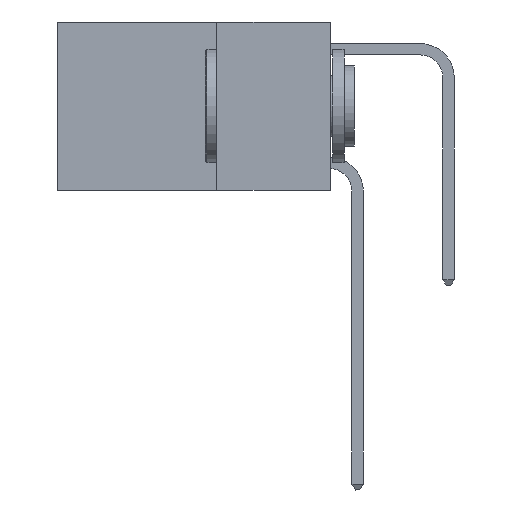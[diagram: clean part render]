
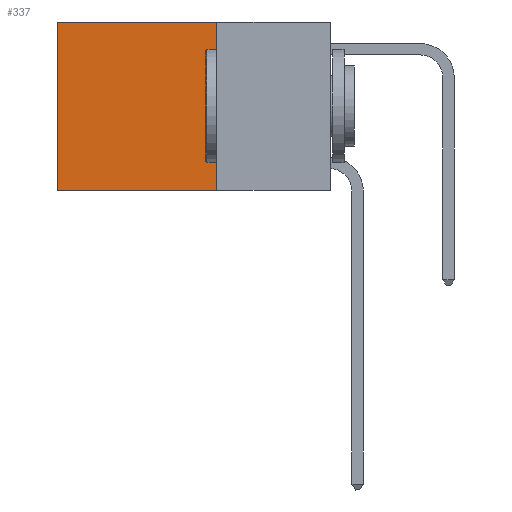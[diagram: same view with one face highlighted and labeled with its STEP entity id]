
A CAD part, left-side view. The second image highlights one B-rep face of the part: STEP entity #337.
In plain terms, the highlighted planar face has unit normal (-1, 0, 0).
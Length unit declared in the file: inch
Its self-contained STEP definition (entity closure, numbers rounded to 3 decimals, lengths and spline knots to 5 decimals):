
#337 = ADVANCED_FACE ( 'NONE', ( #9357 ), #15472, .F. ) ;
#1582 = VECTOR ( 'NONE', #10445, 39.37008 ) ;
#2863 = LINE ( 'NONE', #17177, #15475 ) ;
#3559 = EDGE_CURVE ( 'NONE', #11916, #4300, #12638, .T. ) ;
#3934 = ORIENTED_EDGE ( 'NONE', *, *, #18398, .F. ) ;
#4144 = VERTEX_POINT ( 'NONE', #17875 ) ;
#4300 = VERTEX_POINT ( 'NONE', #13515 ) ;
#6035 = CARTESIAN_POINT ( 'NONE',  ( 0.2625, 0.25, 0. ) ) ;
#6379 = VERTEX_POINT ( 'NONE', #6723 ) ;
#6723 = CARTESIAN_POINT ( 'NONE',  ( 0.2625, 0.25, -0.37 ) ) ;
#7664 = ORIENTED_EDGE ( 'NONE', *, *, #3559, .T. ) ;
#8475 = CARTESIAN_POINT ( 'NONE',  ( 0.2625, 0.25, -0.37 ) ) ;
#9197 = DIRECTION ( 'NONE',  ( 0., 0., -1. ) ) ;
#9357 = FACE_OUTER_BOUND ( 'NONE', #14373, .T. ) ;
#10445 = DIRECTION ( 'NONE',  ( 0., 1., 0. ) ) ;
#10601 = CARTESIAN_POINT ( 'NONE',  ( 0.2625, 0.25, 0. ) ) ;
#11369 = CARTESIAN_POINT ( 'NONE',  ( 0.2625, 0.6, 0. ) ) ;
#11916 = VERTEX_POINT ( 'NONE', #19436 ) ;
#11977 = ORIENTED_EDGE ( 'NONE', *, *, #15067, .T. ) ;
#12050 = DIRECTION ( 'NONE',  ( 0., 1., 0. ) ) ;
#12357 = LINE ( 'NONE', #6035, #20412 ) ;
#12638 = LINE ( 'NONE', #11369, #14411 ) ;
#13515 = CARTESIAN_POINT ( 'NONE',  ( 0.2625, 0.6, -0.37 ) ) ;
#14373 = EDGE_LOOP ( 'NONE', ( #7664, #3934, #14438, #11977 ) ) ;
#14411 = VECTOR ( 'NONE', #15859, 39.37008 ) ;
#14438 = ORIENTED_EDGE ( 'NONE', *, *, #20375, .F. ) ;
#15067 = EDGE_CURVE ( 'NONE', #4144, #11916, #12357, .T. ) ;
#15472 = PLANE ( 'NONE',  #18554 ) ;
#15475 = VECTOR ( 'NONE', #9197, 39.37008 ) ;
#15669 = DIRECTION ( 'NONE',  ( 1., 0., 0. ) ) ;
#15859 = DIRECTION ( 'NONE',  ( 0., 0., -1. ) ) ;
#17177 = CARTESIAN_POINT ( 'NONE',  ( 0.2625, 0.25, 0. ) ) ;
#17875 = CARTESIAN_POINT ( 'NONE',  ( 0.2625, 0.25, 0. ) ) ;
#18398 = EDGE_CURVE ( 'NONE', #6379, #4300, #19472, .T. ) ;
#18554 = AXIS2_PLACEMENT_3D ( 'NONE', #10601, #15669, #18588 ) ;
#18588 = DIRECTION ( 'NONE',  ( 0., 0., -1. ) ) ;
#19436 = CARTESIAN_POINT ( 'NONE',  ( 0.2625, 0.6, 0. ) ) ;
#19472 = LINE ( 'NONE', #8475, #1582 ) ;
#20375 = EDGE_CURVE ( 'NONE', #4144, #6379, #2863, .T. ) ;
#20412 = VECTOR ( 'NONE', #12050, 39.37008 ) ;
